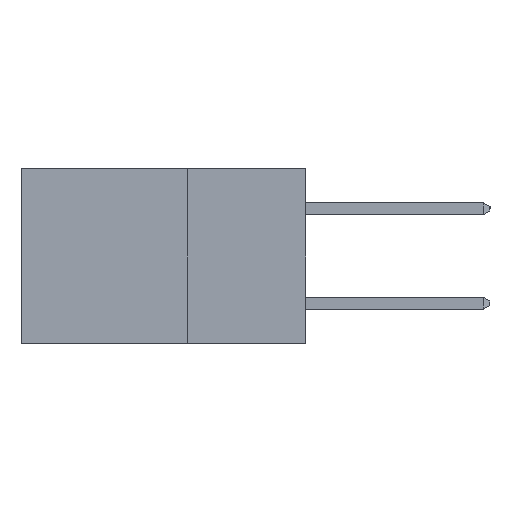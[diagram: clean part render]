
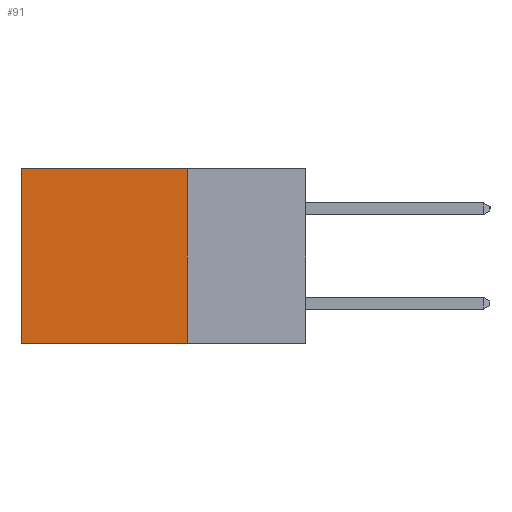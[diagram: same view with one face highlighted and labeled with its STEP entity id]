
A CAD part, left-side view. The second image highlights one B-rep face of the part: STEP entity #91.
In plain terms, the highlighted planar face has unit normal (-1, 0, 0).
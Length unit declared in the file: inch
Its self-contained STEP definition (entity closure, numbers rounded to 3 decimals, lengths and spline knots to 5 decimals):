
#91 = ADVANCED_FACE ( 'NONE', ( #2063 ), #2917, .F. ) ;
#127 = CARTESIAN_POINT ( 'NONE',  ( 0.2615, 0.25, -0.37 ) ) ;
#305 = AXIS2_PLACEMENT_3D ( 'NONE', #3044, #4937, #3996 ) ;
#556 = VECTOR ( 'NONE', #9116, 39.37008 ) ;
#650 = LINE ( 'NONE', #3430, #10940 ) ;
#1634 = VERTEX_POINT ( 'NONE', #5539 ) ;
#1638 = EDGE_CURVE ( 'NONE', #9017, #1634, #650, .T. ) ;
#2063 = FACE_OUTER_BOUND ( 'NONE', #12568, .T. ) ;
#2542 = CARTESIAN_POINT ( 'NONE',  ( 0.2615, 0.6, -0.37 ) ) ;
#2556 = VERTEX_POINT ( 'NONE', #12078 ) ;
#2596 = EDGE_CURVE ( 'NONE', #9017, #2556, #8012, .T. ) ;
#2917 = PLANE ( 'NONE',  #305 ) ;
#2984 = ORIENTED_EDGE ( 'NONE', *, *, #1638, .F. ) ;
#3044 = CARTESIAN_POINT ( 'NONE',  ( 0.2615, 0.25, -0.37 ) ) ;
#3250 = LINE ( 'NONE', #127, #11250 ) ;
#3430 = CARTESIAN_POINT ( 'NONE',  ( 0.2615, 0.25, -0.37 ) ) ;
#3996 = DIRECTION ( 'NONE',  ( 0., 0., -1. ) ) ;
#4085 = LINE ( 'NONE', #6267, #11029 ) ;
#4937 = DIRECTION ( 'NONE',  ( 1., 0., 0. ) ) ;
#5539 = CARTESIAN_POINT ( 'NONE',  ( 0.2615, 0.25, -0.37 ) ) ;
#5553 = ORIENTED_EDGE ( 'NONE', *, *, #2596, .T. ) ;
#6267 = CARTESIAN_POINT ( 'NONE',  ( 0.2615, 0.6, -0.37 ) ) ;
#6961 = EDGE_CURVE ( 'NONE', #1634, #10124, #3250, .T. ) ;
#6962 = EDGE_CURVE ( 'NONE', #2556, #10124, #4085, .T. ) ;
#7129 = CARTESIAN_POINT ( 'NONE',  ( 0.2615, 0.25, 0. ) ) ;
#7940 = ORIENTED_EDGE ( 'NONE', *, *, #6961, .F. ) ;
#8012 = LINE ( 'NONE', #7129, #556 ) ;
#8607 = CARTESIAN_POINT ( 'NONE',  ( 0.2615, 0.25, 0. ) ) ;
#9017 = VERTEX_POINT ( 'NONE', #8607 ) ;
#9099 = DIRECTION ( 'NONE',  ( 0., 1., 0. ) ) ;
#9116 = DIRECTION ( 'NONE',  ( 0., 1., 0. ) ) ;
#10124 = VERTEX_POINT ( 'NONE', #2542 ) ;
#10419 = DIRECTION ( 'NONE',  ( 0., 0., -1. ) ) ;
#10940 = VECTOR ( 'NONE', #10419, 39.37008 ) ;
#11029 = VECTOR ( 'NONE', #11989, 39.37008 ) ;
#11250 = VECTOR ( 'NONE', #9099, 39.37008 ) ;
#11989 = DIRECTION ( 'NONE',  ( 0., 0., -1. ) ) ;
#12066 = ORIENTED_EDGE ( 'NONE', *, *, #6962, .T. ) ;
#12078 = CARTESIAN_POINT ( 'NONE',  ( 0.2615, 0.6, 0. ) ) ;
#12568 = EDGE_LOOP ( 'NONE', ( #12066, #7940, #2984, #5553 ) ) ;
